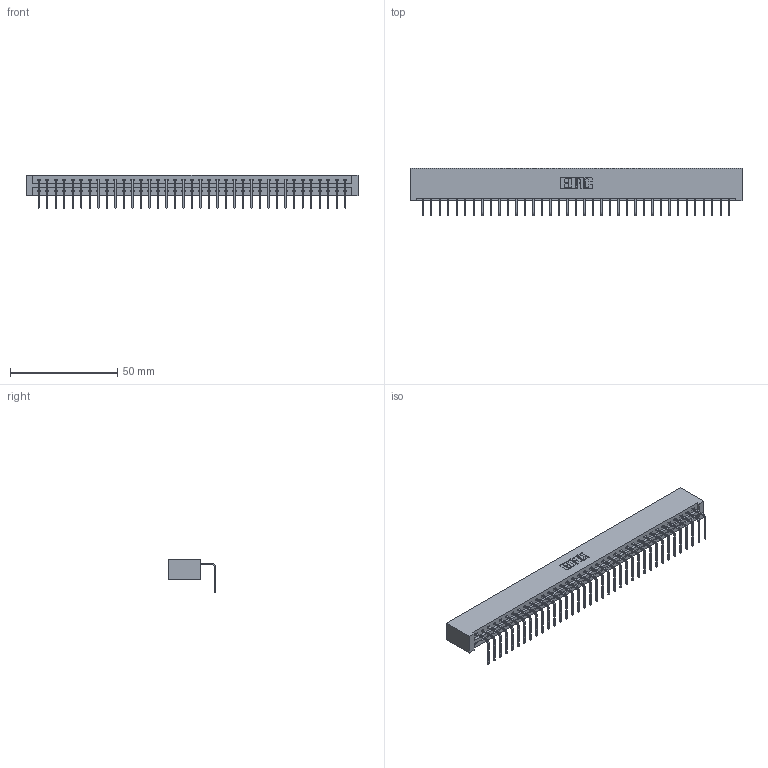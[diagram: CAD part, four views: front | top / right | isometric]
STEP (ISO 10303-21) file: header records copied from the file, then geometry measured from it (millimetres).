
FILE_DESCRIPTION (( 'STEP AP203' ), '1' );
FILE_NAME ('387-037-558-101.STEP', '2019-10-07T20:46:08', ( '' ), ( '' ), 'SwSTEP 2.0', 'SolidWorks 2016', '' );
FILE_SCHEMA (( 'CONFIG_CONTROL_DESIGN' ));
Length unit declared in the file: inch
Products named in the file (3): 337 Part_No Mounting Lugs; 387-037-558-101; 345-292-001_558 Tail - 2
Assembly tree (38 placements, depth 2):
  387-037-558-101
    337 Part_No Mounting Lugs
    345-292-001_558 Tail - 2  x37
Bounding box: 154.48 x 22.17 x 15.37 mm (x, y, z)
Volume: 16855.3 mm3; surface area: 18128.5 mm2
Topology: 38 solids, 38 shells, 2474 faces, 7465 edges, 4926 vertices
Faces by surface type: plane 1842, cylinder 632
Entity records: 27957 total; most frequent: CARTESIAN_POINT 4877, ORIENTED_EDGE 4850, DIRECTION 4107, EDGE_CURVE 2425, LINE 2305, VECTOR 2305, VERTEX_POINT 1614, AXIS2_PLACEMENT_3D 901
